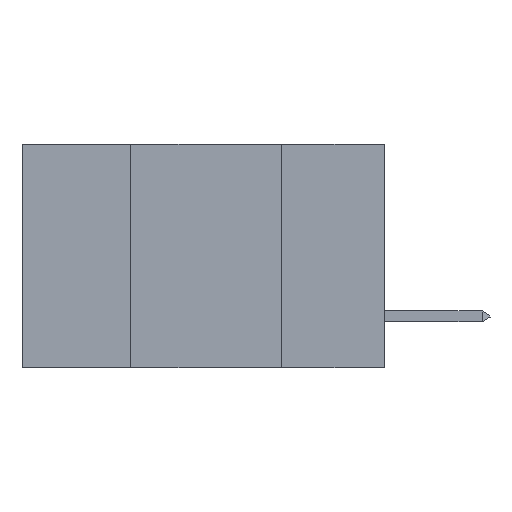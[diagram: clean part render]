
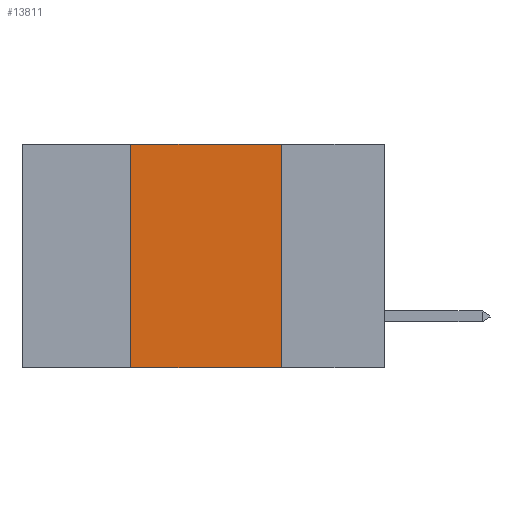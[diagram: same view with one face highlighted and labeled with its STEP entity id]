
A CAD part, left-side view. The second image highlights one B-rep face of the part: STEP entity #13811.
In plain terms, the highlighted planar face has unit normal (-1, 0, 0).
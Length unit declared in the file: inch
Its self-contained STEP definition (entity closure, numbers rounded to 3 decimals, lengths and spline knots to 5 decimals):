
#1611 = CARTESIAN_POINT ( 'NONE',  ( 0., 0.42, 0. ) ) ;
#4338 = DIRECTION ( 'NONE',  ( 0., 0., 1. ) ) ;
#4934 = CARTESIAN_POINT ( 'NONE',  ( 0., 0.6, 0. ) ) ;
#6410 = ORIENTED_EDGE ( 'NONE', *, *, #11944, .F. ) ;
#6973 = CARTESIAN_POINT ( 'NONE',  ( 0., 0.17, 0. ) ) ;
#8852 = LINE ( 'NONE', #21759, #31265 ) ;
#10425 = EDGE_CURVE ( 'NONE', #44463, #39613, #28687, .T. ) ;
#11944 = EDGE_CURVE ( 'NONE', #24094, #44463, #8852, .T. ) ;
#13811 = ADVANCED_FACE ( 'NONE', ( #22446 ), #19117, .F. ) ;
#15329 = CARTESIAN_POINT ( 'NONE',  ( 0., 0.17, -0.37 ) ) ;
#18054 = DIRECTION ( 'NONE',  ( 0., 0., -1. ) ) ;
#18806 = VERTEX_POINT ( 'NONE', #15329 ) ;
#19117 = PLANE ( 'NONE',  #21097 ) ;
#21097 = AXIS2_PLACEMENT_3D ( 'NONE', #4934, #29536, #43481 ) ;
#21480 = ORIENTED_EDGE ( 'NONE', *, *, #10425, .F. ) ;
#21614 = CARTESIAN_POINT ( 'NONE',  ( 0., 0.42, -0.37 ) ) ;
#21759 = CARTESIAN_POINT ( 'NONE',  ( 0., 0.42, 0. ) ) ;
#22446 = FACE_OUTER_BOUND ( 'NONE', #23078, .T. ) ;
#23078 = EDGE_LOOP ( 'NONE', ( #30744, #21480, #6410, #39696 ) ) ;
#24094 = VERTEX_POINT ( 'NONE', #21614 ) ;
#24233 = EDGE_CURVE ( 'NONE', #24094, #18806, #33272, .T. ) ;
#25074 = CARTESIAN_POINT ( 'NONE',  ( 0., 0.17, 0. ) ) ;
#25339 = DIRECTION ( 'NONE',  ( 0., -1., 0. ) ) ;
#25897 = CARTESIAN_POINT ( 'NONE',  ( 0., 0.6, -0.37 ) ) ;
#27022 = VECTOR ( 'NONE', #25339, 39.37008 ) ;
#28289 = LINE ( 'NONE', #25074, #29378 ) ;
#28687 = LINE ( 'NONE', #42669, #27022 ) ;
#29378 = VECTOR ( 'NONE', #18054, 39.37008 ) ;
#29536 = DIRECTION ( 'NONE',  ( 1., 0., 0. ) ) ;
#30744 = ORIENTED_EDGE ( 'NONE', *, *, #42025, .F. ) ;
#31265 = VECTOR ( 'NONE', #4338, 39.37008 ) ;
#31650 = VECTOR ( 'NONE', #33550, 39.37008 ) ;
#33272 = LINE ( 'NONE', #25897, #31650 ) ;
#33550 = DIRECTION ( 'NONE',  ( 0., -1., 0. ) ) ;
#39613 = VERTEX_POINT ( 'NONE', #6973 ) ;
#39696 = ORIENTED_EDGE ( 'NONE', *, *, #24233, .T. ) ;
#42025 = EDGE_CURVE ( 'NONE', #39613, #18806, #28289, .T. ) ;
#42669 = CARTESIAN_POINT ( 'NONE',  ( 0., 0.6, 0. ) ) ;
#43481 = DIRECTION ( 'NONE',  ( 0., 0., -1. ) ) ;
#44463 = VERTEX_POINT ( 'NONE', #1611 ) ;
